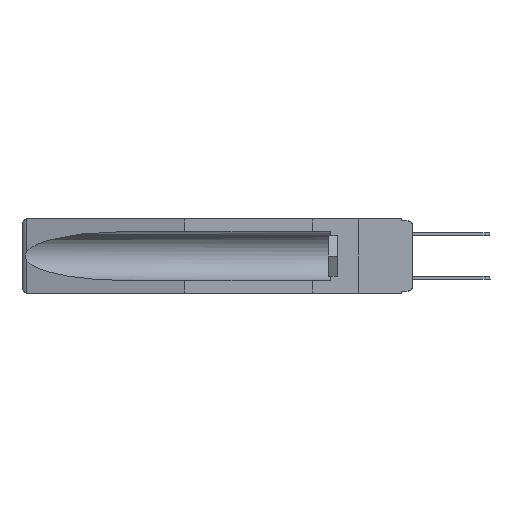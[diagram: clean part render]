
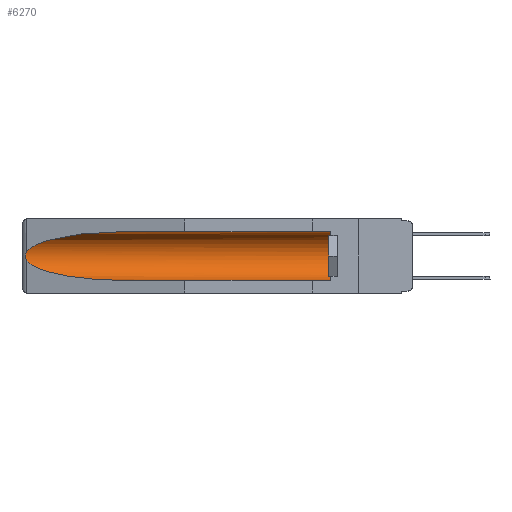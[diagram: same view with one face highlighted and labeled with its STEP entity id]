
A CAD part, left-side view. The second image highlights one B-rep face of the part: STEP entity #6270.
In plain terms, the highlighted cylindrical face has radius 2.857 mm (diameter 5.715 mm), a partial arc.
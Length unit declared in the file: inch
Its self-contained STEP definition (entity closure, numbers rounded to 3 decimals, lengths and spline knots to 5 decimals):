
#709 = EDGE_CURVE ( 'NONE', #12118, #9045, #2673, .T. ) ;
#803 = CARTESIAN_POINT ( 'NONE',  ( 0.155, 0.126, -0.284 ) ) ;
#1485 = CARTESIAN_POINT ( 'NONE',  ( 0.155, 1.07973, -0.059 ) ) ;
#1550 = CARTESIAN_POINT ( 'NONE',  ( 0.26537, 1.52718, -0.19328 ) ) ;
#2271 = LINE ( 'NONE', #21175, #22057 ) ;
#2517 = CARTESIAN_POINT ( 'NONE',  ( 0.26537, 1.52718, -0.14972 ) ) ;
#2673 =( BOUNDED_CURVE ( )  B_SPLINE_CURVE ( 3, ( #1550, #18801, #9157, #17167 ),
 .UNSPECIFIED., .F., .F. ) 
 B_SPLINE_CURVE_WITH_KNOTS ( ( 4, 4 ),
 ( 0.1948, 1.5708 ),
 .UNSPECIFIED. ) 
 CURVE ( )  GEOMETRIC_REPRESENTATION_ITEM ( )  RATIONAL_B_SPLINE_CURVE ( ( 1., 0.848, 0.848, 1. ) ) 
 REPRESENTATION_ITEM ( '' )  );
#3702 = CARTESIAN_POINT ( 'NONE',  ( 0.2675, 1.53308, -0.17534 ) ) ;
#3786 = CARTESIAN_POINT ( 'NONE',  ( 0.26537, 1.52718, -0.19328 ) ) ;
#3852 = VERTEX_POINT ( 'NONE', #24328 ) ;
#4276 = ORIENTED_EDGE ( 'NONE', *, *, #10554, .T. ) ;
#4421 = CARTESIAN_POINT ( 'NONE',  ( 0.21114, 1.30732, -0.059 ) ) ;
#4516 = FACE_OUTER_BOUND ( 'NONE', #11764, .T. ) ;
#4983 = DIRECTION ( 'NONE',  ( 0., 1., 0. ) ) ;
#5692 = CARTESIAN_POINT ( 'NONE',  ( 0.2673, 1.53269, -0.17917 ) ) ;
#5929 = VERTEX_POINT ( 'NONE', #1485 ) ;
#6270 = ADVANCED_FACE ( 'NONE', ( #4516 ), #18222, .F. ) ;
#6786 =( BOUNDED_CURVE ( )  B_SPLINE_CURVE ( 3, ( #23874, #4421, #8341, #2517 ),
 .UNSPECIFIED., .F., .F. ) 
 B_SPLINE_CURVE_WITH_KNOTS ( ( 4, 4 ),
 ( 4.71239, 6.08839 ),
 .UNSPECIFIED. ) 
 CURVE ( )  GEOMETRIC_REPRESENTATION_ITEM ( )  RATIONAL_B_SPLINE_CURVE ( ( 1., 0.848, 0.848, 1. ) ) 
 REPRESENTATION_ITEM ( '' )  );
#6902 = AXIS2_PLACEMENT_3D ( 'NONE', #7570, #19132, #16923 ) ;
#7570 = CARTESIAN_POINT ( 'NONE',  ( 0.155, 0.126, -0.1715 ) ) ;
#8341 = CARTESIAN_POINT ( 'NONE',  ( 0.25451, 1.48313, -0.09465 ) ) ;
#8928 = LINE ( 'NONE', #18179, #19905 ) ;
#9003 = ORIENTED_EDGE ( 'NONE', *, *, #14412, .T. ) ;
#9045 = VERTEX_POINT ( 'NONE', #12138 ) ;
#9157 = CARTESIAN_POINT ( 'NONE',  ( 0.21114, 1.30732, -0.284 ) ) ;
#9560 = CARTESIAN_POINT ( 'NONE',  ( 0.2673, 1.5327, -0.16383 ) ) ;
#10475 = CARTESIAN_POINT ( 'NONE',  ( 0.155, -0.30754, -0.1715 ) ) ;
#10512 = ORIENTED_EDGE ( 'NONE', *, *, #18455, .F. ) ;
#10554 = EDGE_CURVE ( 'NONE', #13062, #3852, #24729, .T. ) ;
#11505 = CARTESIAN_POINT ( 'NONE',  ( 0.26655, 1.53094, -0.18657 ) ) ;
#11764 = EDGE_LOOP ( 'NONE', ( #16313, #23082, #20070, #10512, #4276, #9003 ) ) ;
#12118 = VERTEX_POINT ( 'NONE', #24375 ) ;
#12138 = CARTESIAN_POINT ( 'NONE',  ( 0.155, 1.07973, -0.284 ) ) ;
#13062 = VERTEX_POINT ( 'NONE', #803 ) ;
#13333 = DIRECTION ( 'NONE',  ( 0., 1., 0. ) ) ;
#13398 = CARTESIAN_POINT ( 'NONE',  ( 0.26597, 1.52961, -0.15275 ) ) ;
#14412 = EDGE_CURVE ( 'NONE', #3852, #5929, #8928, .T. ) ;
#14973 = EDGE_CURVE ( 'NONE', #5929, #22398, #6786, .T. ) ;
#15267 = CARTESIAN_POINT ( 'NONE',  ( 0.26537, 1.52718, -0.14972 ) ) ;
#16313 = ORIENTED_EDGE ( 'NONE', *, *, #14973, .T. ) ;
#16923 = DIRECTION ( 'NONE',  ( 0., 0., 1. ) ) ;
#17167 = CARTESIAN_POINT ( 'NONE',  ( 0.155, 1.07973, -0.284 ) ) ;
#17591 = CARTESIAN_POINT ( 'NONE',  ( 0.2675, 1.53308, -0.16763 ) ) ;
#18179 = CARTESIAN_POINT ( 'NONE',  ( 0.155, -0.30754, -0.059 ) ) ;
#18191 = CARTESIAN_POINT ( 'NONE',  ( 0.26537, 1.52718, -0.14972 ) ) ;
#18222 = CYLINDRICAL_SURFACE ( 'NONE', #23034, 0.1125 ) ;
#18455 = EDGE_CURVE ( 'NONE', #13062, #9045, #2271, .T. ) ;
#18514 = DIRECTION ( 'NONE',  ( 0., 0., 1. ) ) ;
#18801 = CARTESIAN_POINT ( 'NONE',  ( 0.25451, 1.48313, -0.24835 ) ) ;
#19132 = DIRECTION ( 'NONE',  ( 0., -1., 0. ) ) ;
#19370 = CARTESIAN_POINT ( 'NONE',  ( 0.26597, 1.5296, -0.19026 ) ) ;
#19905 = VECTOR ( 'NONE', #21797, 39.37008 ) ;
#20034 = B_SPLINE_CURVE_WITH_KNOTS ( 'NONE', 3,
 ( #15267, #13398, #23410, #9560, #17591, #3702, #5692, #11505, #19370, #3786 ),
 .UNSPECIFIED., .F., .F.,
 ( 4, 2, 2, 2, 4 ),
 ( 0., 0.00029, 0.00058, 0.00087, 0.00117 ),
 .UNSPECIFIED. ) ;
#20070 = ORIENTED_EDGE ( 'NONE', *, *, #709, .T. ) ;
#20291 = EDGE_CURVE ( 'NONE', #22398, #12118, #20034, .T. ) ;
#21175 = CARTESIAN_POINT ( 'NONE',  ( 0.155, -0.30754, -0.284 ) ) ;
#21797 = DIRECTION ( 'NONE',  ( 0., 1., 0. ) ) ;
#22057 = VECTOR ( 'NONE', #13333, 39.37008 ) ;
#22398 = VERTEX_POINT ( 'NONE', #18191 ) ;
#23034 = AXIS2_PLACEMENT_3D ( 'NONE', #10475, #4983, #18514 ) ;
#23082 = ORIENTED_EDGE ( 'NONE', *, *, #20291, .T. ) ;
#23410 = CARTESIAN_POINT ( 'NONE',  ( 0.26654, 1.53092, -0.15636 ) ) ;
#23874 = CARTESIAN_POINT ( 'NONE',  ( 0.155, 1.07973, -0.059 ) ) ;
#24328 = CARTESIAN_POINT ( 'NONE',  ( 0.155, 0.126, -0.059 ) ) ;
#24375 = CARTESIAN_POINT ( 'NONE',  ( 0.26537, 1.52718, -0.19328 ) ) ;
#24729 = CIRCLE ( 'NONE', #6902, 0.1125 ) ;
